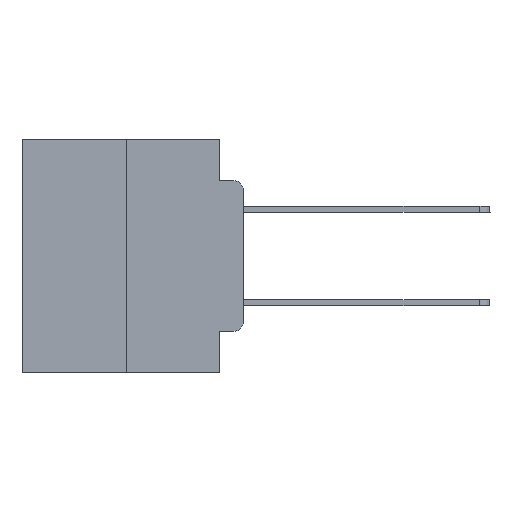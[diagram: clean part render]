
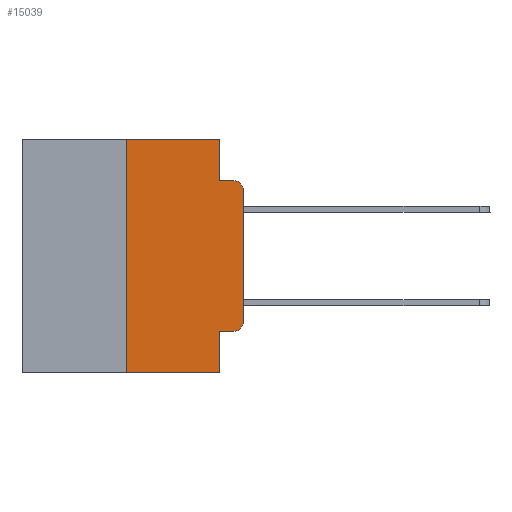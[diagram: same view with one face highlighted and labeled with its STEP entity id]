
A CAD part, left-side view. The second image highlights one B-rep face of the part: STEP entity #15039.
In plain terms, the highlighted planar face has unit normal (-1, 0, 0).
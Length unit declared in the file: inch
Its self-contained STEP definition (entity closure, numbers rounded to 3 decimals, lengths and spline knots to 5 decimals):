
#322 = CIRCLE ( 'NONE', #18534, 0.02 ) ;
#354 = DIRECTION ( 'NONE',  ( 0., 0., -1. ) ) ;
#451 = CARTESIAN_POINT ( 'NONE',  ( 0., 0.051, -0.4115 ) ) ;
#524 = DIRECTION ( 'NONE',  ( 1., 0., 0. ) ) ;
#685 = CARTESIAN_POINT ( 'NONE',  ( 0., 0.02, -0.3915 ) ) ;
#733 = EDGE_CURVE ( 'NONE', #27350, #23820, #16873, .T. ) ;
#847 = VERTEX_POINT ( 'NONE', #2181 ) ;
#1129 = ORIENTED_EDGE ( 'NONE', *, *, #12759, .F. ) ;
#1157 = EDGE_CURVE ( 'NONE', #13412, #26108, #6800, .T. ) ;
#1417 = VERTEX_POINT ( 'NONE', #15504 ) ;
#1480 = DIRECTION ( 'NONE',  ( 0., -1., 0. ) ) ;
#2181 = CARTESIAN_POINT ( 'NONE',  ( 0., 0.02, -0.4115 ) ) ;
#3853 = CARTESIAN_POINT ( 'NONE',  ( 0., 0.051, -0.0885 ) ) ;
#4095 = ORIENTED_EDGE ( 'NONE', *, *, #5111, .T. ) ;
#4286 = AXIS2_PLACEMENT_3D ( 'NONE', #27131, #524, #11589 ) ;
#4705 = DIRECTION ( 'NONE',  ( 0., -1., 0. ) ) ;
#4922 = DIRECTION ( 'NONE',  ( -1., 0., 0. ) ) ;
#4937 = VERTEX_POINT ( 'NONE', #13805 ) ;
#5111 = EDGE_CURVE ( 'NONE', #847, #1417, #322, .T. ) ;
#5247 = DIRECTION ( 'NONE',  ( 0., 0., -1. ) ) ;
#5725 = CARTESIAN_POINT ( 'NONE',  ( 0., 0.02, -0.0885 ) ) ;
#6431 = VERTEX_POINT ( 'NONE', #8295 ) ;
#6516 = ORIENTED_EDGE ( 'NONE', *, *, #14889, .T. ) ;
#6800 = LINE ( 'NONE', #10382, #26128 ) ;
#6861 = VERTEX_POINT ( 'NONE', #14835 ) ;
#7454 = VECTOR ( 'NONE', #5247, 39.37008 ) ;
#8295 = CARTESIAN_POINT ( 'NONE',  ( 0., 0.051, -0.4115 ) ) ;
#8489 = CIRCLE ( 'NONE', #16710, 0.02 ) ;
#8560 = ORIENTED_EDGE ( 'NONE', *, *, #11766, .T. ) ;
#10048 = ORIENTED_EDGE ( 'NONE', *, *, #22296, .F. ) ;
#10289 = DIRECTION ( 'NONE',  ( 0., 0., 1. ) ) ;
#10382 = CARTESIAN_POINT ( 'NONE',  ( 0., 0.25, 0. ) ) ;
#10541 = CARTESIAN_POINT ( 'NONE',  ( 0., 0.473, 0. ) ) ;
#10594 = VECTOR ( 'NONE', #354, 39.37008 ) ;
#10668 = CARTESIAN_POINT ( 'NONE',  ( 0., 0.051, -0.0885 ) ) ;
#11589 = DIRECTION ( 'NONE',  ( 0., 0., -1. ) ) ;
#11766 = EDGE_CURVE ( 'NONE', #1417, #6861, #14866, .T. ) ;
#12348 = LINE ( 'NONE', #19126, #23426 ) ;
#12714 = CARTESIAN_POINT ( 'NONE',  ( 0., 0., 0. ) ) ;
#12759 = EDGE_CURVE ( 'NONE', #23820, #23042, #23099, .T. ) ;
#12929 = DIRECTION ( 'NONE',  ( 0., -1., 0. ) ) ;
#13096 = EDGE_CURVE ( 'NONE', #13412, #4937, #12348, .T. ) ;
#13360 = DIRECTION ( 'NONE',  ( 0., 0., -1. ) ) ;
#13412 = VERTEX_POINT ( 'NONE', #28523 ) ;
#13455 = ORIENTED_EDGE ( 'NONE', *, *, #20863, .F. ) ;
#13805 = CARTESIAN_POINT ( 'NONE',  ( 0., 0.051, -0.5 ) ) ;
#14019 = CARTESIAN_POINT ( 'NONE',  ( 0., 0.051, 0. ) ) ;
#14558 = DIRECTION ( 'NONE',  ( 0., 0., 1. ) ) ;
#14752 = ORIENTED_EDGE ( 'NONE', *, *, #13096, .T. ) ;
#14835 = CARTESIAN_POINT ( 'NONE',  ( 0., 0., -0.1085 ) ) ;
#14866 = LINE ( 'NONE', #12714, #19702 ) ;
#14889 = EDGE_CURVE ( 'NONE', #6861, #23042, #8489, .T. ) ;
#15039 = ADVANCED_FACE ( 'NONE', ( #19550 ), #22638, .F. ) ;
#15504 = CARTESIAN_POINT ( 'NONE',  ( 0., 0., -0.3915 ) ) ;
#15867 = LINE ( 'NONE', #10541, #21062 ) ;
#16710 = AXIS2_PLACEMENT_3D ( 'NONE', #24359, #26748, #13360 ) ;
#16827 = LINE ( 'NONE', #26770, #10594 ) ;
#16873 = LINE ( 'NONE', #14019, #7454 ) ;
#18534 = AXIS2_PLACEMENT_3D ( 'NONE', #685, #4922, #27187 ) ;
#18877 = VECTOR ( 'NONE', #4705, 39.37008 ) ;
#18972 = VECTOR ( 'NONE', #24150, 39.37008 ) ;
#19108 = ORIENTED_EDGE ( 'NONE', *, *, #1157, .F. ) ;
#19126 = CARTESIAN_POINT ( 'NONE',  ( 0., 0.473, -0.5 ) ) ;
#19550 = FACE_OUTER_BOUND ( 'NONE', #26945, .T. ) ;
#19702 = VECTOR ( 'NONE', #14558, 39.37008 ) ;
#20602 = LINE ( 'NONE', #451, #18877 ) ;
#20863 = EDGE_CURVE ( 'NONE', #26108, #27350, #15867, .T. ) ;
#21062 = VECTOR ( 'NONE', #12929, 39.37008 ) ;
#22214 = EDGE_CURVE ( 'NONE', #6431, #847, #20602, .T. ) ;
#22296 = EDGE_CURVE ( 'NONE', #6431, #4937, #16827, .T. ) ;
#22506 = ORIENTED_EDGE ( 'NONE', *, *, #733, .F. ) ;
#22638 = PLANE ( 'NONE',  #4286 ) ;
#22930 = CARTESIAN_POINT ( 'NONE',  ( 0., 0.25, 0. ) ) ;
#23042 = VERTEX_POINT ( 'NONE', #5725 ) ;
#23099 = LINE ( 'NONE', #10668, #18972 ) ;
#23426 = VECTOR ( 'NONE', #1480, 39.37008 ) ;
#23820 = VERTEX_POINT ( 'NONE', #3853 ) ;
#24150 = DIRECTION ( 'NONE',  ( 0., -1., 0. ) ) ;
#24359 = CARTESIAN_POINT ( 'NONE',  ( 0., 0.02, -0.1085 ) ) ;
#25614 = CARTESIAN_POINT ( 'NONE',  ( 0., 0.051, 0. ) ) ;
#26108 = VERTEX_POINT ( 'NONE', #22930 ) ;
#26128 = VECTOR ( 'NONE', #10289, 39.37008 ) ;
#26625 = ORIENTED_EDGE ( 'NONE', *, *, #22214, .T. ) ;
#26748 = DIRECTION ( 'NONE',  ( -1., 0., 0. ) ) ;
#26770 = CARTESIAN_POINT ( 'NONE',  ( 0., 0.051, 0. ) ) ;
#26945 = EDGE_LOOP ( 'NONE', ( #8560, #6516, #1129, #22506, #13455, #19108, #14752, #10048, #26625, #4095 ) ) ;
#27131 = CARTESIAN_POINT ( 'NONE',  ( 0., 0.473, 0. ) ) ;
#27187 = DIRECTION ( 'NONE',  ( 0., 0., -1. ) ) ;
#27350 = VERTEX_POINT ( 'NONE', #25614 ) ;
#28523 = CARTESIAN_POINT ( 'NONE',  ( 0., 0.25, -0.5 ) ) ;
